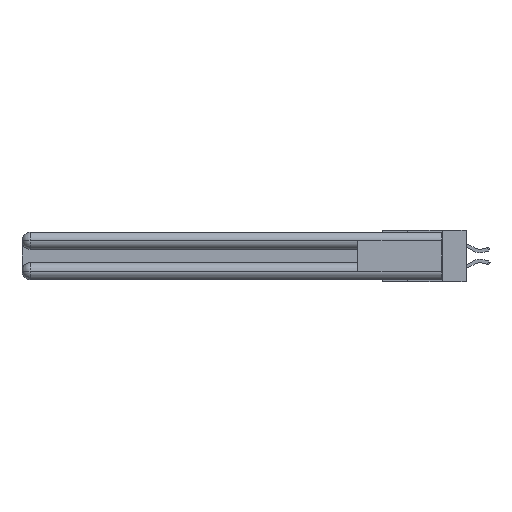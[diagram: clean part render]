
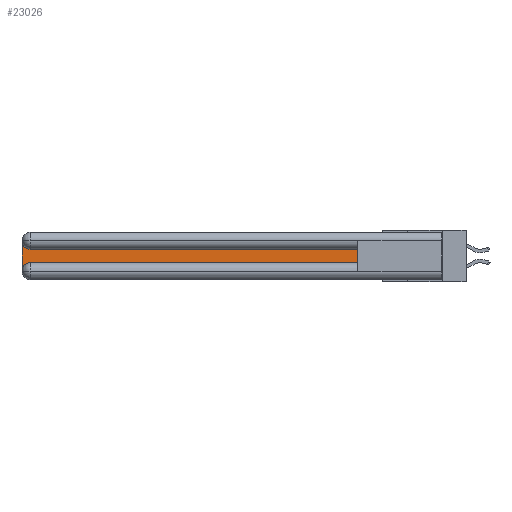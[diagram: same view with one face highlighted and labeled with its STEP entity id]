
A CAD part, left-side view. The second image highlights one B-rep face of the part: STEP entity #23026.
In plain terms, the highlighted planar face has unit normal (-1, 0, 0).
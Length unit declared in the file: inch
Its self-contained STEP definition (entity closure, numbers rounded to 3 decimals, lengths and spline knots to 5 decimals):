
#892 = LINE ( 'NONE', #30273, #22339 ) ;
#930 = DIRECTION ( 'NONE',  ( 1., 0., 0. ) ) ;
#2265 = ORIENTED_EDGE ( 'NONE', *, *, #17903, .T. ) ;
#2322 = EDGE_CURVE ( 'NONE', #29529, #29337, #16217, .T. ) ;
#2541 = EDGE_CURVE ( 'NONE', #21405, #29529, #16639, .T. ) ;
#2708 = ORIENTED_EDGE ( 'NONE', *, *, #26468, .T. ) ;
#4177 = AXIS2_PLACEMENT_3D ( 'NONE', #17572, #930, #26239 ) ;
#5679 = VERTEX_POINT ( 'NONE', #16219 ) ;
#6918 = CARTESIAN_POINT ( 'NONE',  ( 0.075, 2.94, -0.2175 ) ) ;
#8068 = DIRECTION ( 'NONE',  ( 0., -1., 0. ) ) ;
#10177 = DIRECTION ( 'NONE',  ( 0., 0., -1. ) ) ;
#10817 = ORIENTED_EDGE ( 'NONE', *, *, #2322, .T. ) ;
#10897 = DIRECTION ( 'NONE',  ( 0., 1., 0. ) ) ;
#11316 = AXIS2_PLACEMENT_3D ( 'NONE', #30267, #19006, #10177 ) ;
#15955 = CARTESIAN_POINT ( 'NONE',  ( 0.075, 3., -0.1225 ) ) ;
#16217 = CIRCLE ( 'NONE', #4177, 0.06 ) ;
#16219 = CARTESIAN_POINT ( 'NONE',  ( 0.075, 0.6, -0.1225 ) ) ;
#16639 = LINE ( 'NONE', #35321, #32848 ) ;
#17292 = DIRECTION ( 'NONE',  ( 0., 0., 1. ) ) ;
#17572 = CARTESIAN_POINT ( 'NONE',  ( 0.075, 2.94, -0.2775 ) ) ;
#17903 = EDGE_CURVE ( 'NONE', #30735, #21405, #28680, .T. ) ;
#19006 = DIRECTION ( 'NONE',  ( 1., 0., 0. ) ) ;
#19712 = ORIENTED_EDGE ( 'NONE', *, *, #27855, .T. ) ;
#19882 = CARTESIAN_POINT ( 'NONE',  ( 0.075, 3., -0.0625 ) ) ;
#21046 = CARTESIAN_POINT ( 'NONE',  ( 0.075, 0.6, -0.2175 ) ) ;
#21405 = VERTEX_POINT ( 'NONE', #19882 ) ;
#22026 = DIRECTION ( 'NONE',  ( 0., 0., -1. ) ) ;
#22339 = VECTOR ( 'NONE', #17292, 39.37008 ) ;
#22340 = CARTESIAN_POINT ( 'NONE',  ( 0.075, 2.94, -0.1225 ) ) ;
#23026 = ADVANCED_FACE ( 'NONE', ( #29300 ), #32728, .F. ) ;
#23788 = LINE ( 'NONE', #26705, #26829 ) ;
#24071 = CARTESIAN_POINT ( 'NONE',  ( 0.075, 3., -0.2775 ) ) ;
#24133 = VERTEX_POINT ( 'NONE', #27784 ) ;
#24251 = EDGE_CURVE ( 'NONE', #29337, #24133, #29194, .T. ) ;
#24382 = DIRECTION ( 'NONE',  ( 1., 0., 0. ) ) ;
#25443 = ORIENTED_EDGE ( 'NONE', *, *, #24251, .T. ) ;
#26239 = DIRECTION ( 'NONE',  ( 0., 0., -1. ) ) ;
#26468 = EDGE_CURVE ( 'NONE', #5679, #30735, #23788, .T. ) ;
#26705 = CARTESIAN_POINT ( 'NONE',  ( 0.075, 0.6, -0.1225 ) ) ;
#26829 = VECTOR ( 'NONE', #10897, 39.37008 ) ;
#27611 = EDGE_LOOP ( 'NONE', ( #2708, #2265, #28249, #10817, #25443, #19712 ) ) ;
#27784 = CARTESIAN_POINT ( 'NONE',  ( 0.075, 0.6, -0.2175 ) ) ;
#27855 = EDGE_CURVE ( 'NONE', #24133, #5679, #892, .T. ) ;
#28249 = ORIENTED_EDGE ( 'NONE', *, *, #2541, .T. ) ;
#28680 = CIRCLE ( 'NONE', #11316, 0.06 ) ;
#29194 = LINE ( 'NONE', #21046, #34044 ) ;
#29300 = FACE_OUTER_BOUND ( 'NONE', #27611, .T. ) ;
#29337 = VERTEX_POINT ( 'NONE', #6918 ) ;
#29529 = VERTEX_POINT ( 'NONE', #24071 ) ;
#30267 = CARTESIAN_POINT ( 'NONE',  ( 0.075, 2.94, -0.0625 ) ) ;
#30273 = CARTESIAN_POINT ( 'NONE',  ( 0.075, 0.6, -0.2175 ) ) ;
#30735 = VERTEX_POINT ( 'NONE', #22340 ) ;
#32728 = PLANE ( 'NONE',  #33042 ) ;
#32848 = VECTOR ( 'NONE', #35811, 39.37008 ) ;
#33042 = AXIS2_PLACEMENT_3D ( 'NONE', #15955, #24382, #22026 ) ;
#34044 = VECTOR ( 'NONE', #8068, 39.37008 ) ;
#35321 = CARTESIAN_POINT ( 'NONE',  ( 0.075, 3., -0.2175 ) ) ;
#35811 = DIRECTION ( 'NONE',  ( 0., 0., -1. ) ) ;
